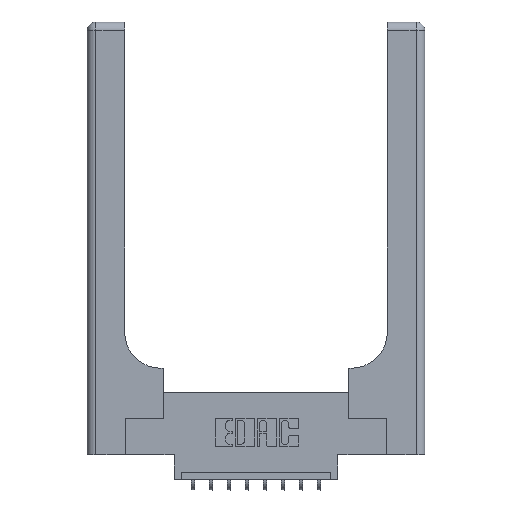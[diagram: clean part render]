
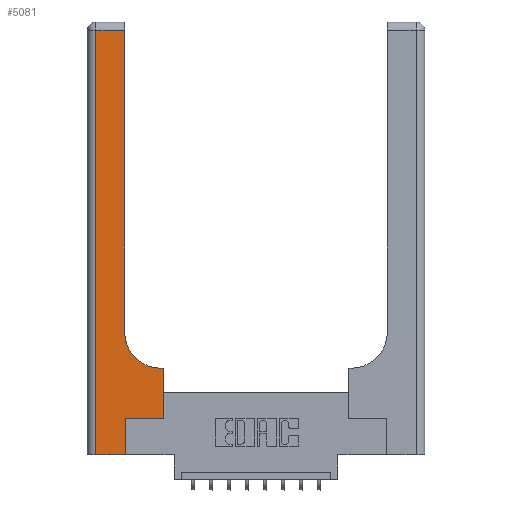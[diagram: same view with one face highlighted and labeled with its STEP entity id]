
A CAD part, top view. The second image highlights one B-rep face of the part: STEP entity #5081.
In plain terms, the highlighted planar face has unit normal (0, 0, 1).
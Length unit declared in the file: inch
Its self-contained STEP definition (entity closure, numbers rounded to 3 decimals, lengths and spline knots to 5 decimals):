
#146 = DIRECTION ( 'NONE',  ( 0., 0., -1. ) ) ;
#317 = VERTEX_POINT ( 'NONE', #5582 ) ;
#408 = EDGE_CURVE ( 'NONE', #9239, #13550, #699, .T. ) ;
#589 = ORIENTED_EDGE ( 'NONE', *, *, #4588, .T. ) ;
#699 = CIRCLE ( 'NONE', #13398, 0.25 ) ;
#965 = VECTOR ( 'NONE', #1342, 39.37008 ) ;
#1342 = DIRECTION ( 'NONE',  ( 0., 1., 0. ) ) ;
#1595 = DIRECTION ( 'NONE',  ( -1., 0., 0. ) ) ;
#1926 = CARTESIAN_POINT ( 'NONE',  ( 0.265, 0., 0.37 ) ) ;
#2010 = ORIENTED_EDGE ( 'NONE', *, *, #7528, .T. ) ;
#2058 = EDGE_CURVE ( 'NONE', #13851, #13136, #6929, .T. ) ;
#2428 = CARTESIAN_POINT ( 'NONE',  ( 0.528, 0.25, 0.37 ) ) ;
#2432 = ORIENTED_EDGE ( 'NONE', *, *, #14634, .T. ) ;
#2710 = LINE ( 'NONE', #13480, #12200 ) ;
#3145 = EDGE_CURVE ( 'NONE', #14061, #9239, #3279, .T. ) ;
#3279 = LINE ( 'NONE', #4205, #14194 ) ;
#3525 = CARTESIAN_POINT ( 'NONE',  ( 0.26, 0.85, 0.37 ) ) ;
#3633 = CARTESIAN_POINT ( 'NONE',  ( 0.265, 0., 0.37 ) ) ;
#4205 = CARTESIAN_POINT ( 'NONE',  ( 0.26, 0.6, 0.37 ) ) ;
#4463 = VECTOR ( 'NONE', #5761, 39.37008 ) ;
#4588 = EDGE_CURVE ( 'NONE', #13550, #317, #9978, .T. ) ;
#5081 = ADVANCED_FACE ( 'NONE', ( #10007 ), #14586, .F. ) ;
#5122 = DIRECTION ( 'NONE',  ( 1., 0., 0. ) ) ;
#5581 = VECTOR ( 'NONE', #11044, 39.37008 ) ;
#5582 = CARTESIAN_POINT ( 'NONE',  ( 0.26, 2.94, 0.37 ) ) ;
#5638 = VECTOR ( 'NONE', #13534, 39.37008 ) ;
#5672 = ORIENTED_EDGE ( 'NONE', *, *, #2058, .T. ) ;
#5761 = DIRECTION ( 'NONE',  ( 1., 0., 0. ) ) ;
#6092 = EDGE_CURVE ( 'NONE', #8877, #14015, #2710, .T. ) ;
#6264 = LINE ( 'NONE', #13467, #5581 ) ;
#6465 = ORIENTED_EDGE ( 'NONE', *, *, #408, .T. ) ;
#6526 = CARTESIAN_POINT ( 'NONE',  ( 0.26, 3., 0.37 ) ) ;
#6697 = DIRECTION ( 'NONE',  ( -1., 0., 0. ) ) ;
#6929 = LINE ( 'NONE', #11688, #4463 ) ;
#7369 = CARTESIAN_POINT ( 'NONE',  ( 0.51, 0.85, 0.37 ) ) ;
#7511 = VECTOR ( 'NONE', #11072, 39.37008 ) ;
#7516 = CARTESIAN_POINT ( 'NONE',  ( 0., 3., 0.37 ) ) ;
#7528 = EDGE_CURVE ( 'NONE', #317, #11697, #6264, .T. ) ;
#7670 = LINE ( 'NONE', #14987, #5638 ) ;
#8035 = AXIS2_PLACEMENT_3D ( 'NONE', #7516, #14814, #1595 ) ;
#8877 = VERTEX_POINT ( 'NONE', #11113 ) ;
#8933 = EDGE_CURVE ( 'NONE', #11697, #8877, #7670, .T. ) ;
#9239 = VERTEX_POINT ( 'NONE', #11944 ) ;
#9349 = ORIENTED_EDGE ( 'NONE', *, *, #15181, .T. ) ;
#9727 = CARTESIAN_POINT ( 'NONE',  ( 0.528, 0.6, 0.37 ) ) ;
#9978 = LINE ( 'NONE', #6526, #7511 ) ;
#10007 = FACE_OUTER_BOUND ( 'NONE', #12605, .T. ) ;
#10102 = CARTESIAN_POINT ( 'NONE',  ( 0.06, 2.94, 0.37 ) ) ;
#10187 = LINE ( 'NONE', #1926, #14068 ) ;
#10261 = DIRECTION ( 'NONE',  ( 0., 1., 0. ) ) ;
#10620 = LINE ( 'NONE', #2428, #965 ) ;
#11039 = DIRECTION ( 'NONE',  ( 1., 0., 0. ) ) ;
#11044 = DIRECTION ( 'NONE',  ( -1., 0., 0. ) ) ;
#11072 = DIRECTION ( 'NONE',  ( 0., 1., 0. ) ) ;
#11113 = CARTESIAN_POINT ( 'NONE',  ( 0.06, 0., 0.37 ) ) ;
#11688 = CARTESIAN_POINT ( 'NONE',  ( 0.265, 0.25, 0.37 ) ) ;
#11697 = VERTEX_POINT ( 'NONE', #10102 ) ;
#11944 = CARTESIAN_POINT ( 'NONE',  ( 0.51, 0.6, 0.37 ) ) ;
#12200 = VECTOR ( 'NONE', #5122, 39.37008 ) ;
#12605 = EDGE_LOOP ( 'NONE', ( #589, #2010, #13423, #14912, #2432, #5672, #9349, #15178, #6465 ) ) ;
#13136 = VERTEX_POINT ( 'NONE', #13154 ) ;
#13154 = CARTESIAN_POINT ( 'NONE',  ( 0.528, 0.25, 0.37 ) ) ;
#13398 = AXIS2_PLACEMENT_3D ( 'NONE', #7369, #146, #11039 ) ;
#13423 = ORIENTED_EDGE ( 'NONE', *, *, #8933, .T. ) ;
#13467 = CARTESIAN_POINT ( 'NONE',  ( 0., 2.94, 0.37 ) ) ;
#13480 = CARTESIAN_POINT ( 'NONE',  ( 0., 0., 0.37 ) ) ;
#13534 = DIRECTION ( 'NONE',  ( 0., -1., 0. ) ) ;
#13550 = VERTEX_POINT ( 'NONE', #3525 ) ;
#13851 = VERTEX_POINT ( 'NONE', #14176 ) ;
#14015 = VERTEX_POINT ( 'NONE', #3633 ) ;
#14061 = VERTEX_POINT ( 'NONE', #9727 ) ;
#14068 = VECTOR ( 'NONE', #10261, 39.37008 ) ;
#14176 = CARTESIAN_POINT ( 'NONE',  ( 0.265, 0.25, 0.37 ) ) ;
#14194 = VECTOR ( 'NONE', #6697, 39.37008 ) ;
#14586 = PLANE ( 'NONE',  #8035 ) ;
#14634 = EDGE_CURVE ( 'NONE', #14015, #13851, #10187, .T. ) ;
#14814 = DIRECTION ( 'NONE',  ( 0., 0., -1. ) ) ;
#14912 = ORIENTED_EDGE ( 'NONE', *, *, #6092, .T. ) ;
#14987 = CARTESIAN_POINT ( 'NONE',  ( 0.06, 3., 0.37 ) ) ;
#15178 = ORIENTED_EDGE ( 'NONE', *, *, #3145, .T. ) ;
#15181 = EDGE_CURVE ( 'NONE', #13136, #14061, #10620, .T. ) ;
